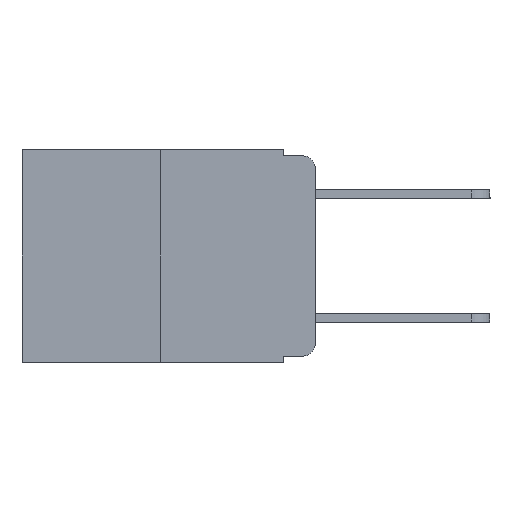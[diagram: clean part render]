
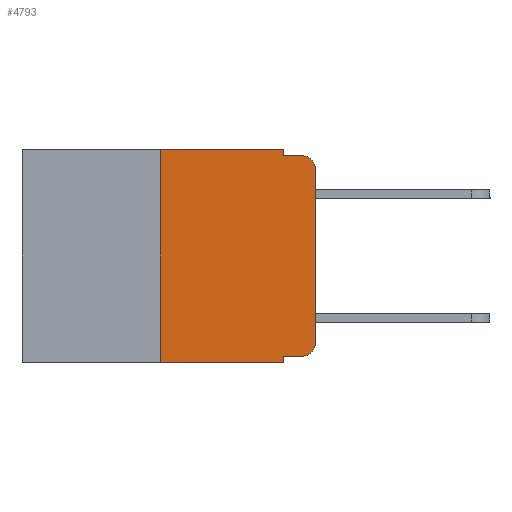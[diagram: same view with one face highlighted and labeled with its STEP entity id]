
A CAD part, left-side view. The second image highlights one B-rep face of the part: STEP entity #4793.
In plain terms, the highlighted planar face has unit normal (-1, 0, 0).
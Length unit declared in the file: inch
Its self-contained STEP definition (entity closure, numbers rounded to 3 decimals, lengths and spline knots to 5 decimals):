
#39 = VERTEX_POINT ( 'NONE', #19924 ) ;
#89 = CARTESIAN_POINT ( 'NONE',  ( 0., 0.473, 0. ) ) ;
#258 = CARTESIAN_POINT ( 'NONE',  ( 0., 0., -0.03 ) ) ;
#409 = PLANE ( 'NONE',  #3439 ) ;
#651 = CARTESIAN_POINT ( 'NONE',  ( 0., 0.473, 0. ) ) ;
#1153 = VERTEX_POINT ( 'NONE', #19772 ) ;
#1173 = ORIENTED_EDGE ( 'NONE', *, *, #15919, .F. ) ;
#1188 = VECTOR ( 'NONE', #7753, 39.37008 ) ;
#1391 = VERTEX_POINT ( 'NONE', #6716 ) ;
#1683 = DIRECTION ( 'NONE',  ( 0., 0., -1. ) ) ;
#2019 = VERTEX_POINT ( 'NONE', #19199 ) ;
#2076 = LINE ( 'NONE', #18464, #6867 ) ;
#2133 = CARTESIAN_POINT ( 'NONE',  ( 0., 0.051, 0. ) ) ;
#2309 = VECTOR ( 'NONE', #15139, 39.37008 ) ;
#2660 = CARTESIAN_POINT ( 'NONE',  ( 0., 0.051, -0.343 ) ) ;
#2833 = AXIS2_PLACEMENT_3D ( 'NONE', #19030, #16500, #13619 ) ;
#2994 = EDGE_CURVE ( 'NONE', #5129, #16042, #19267, .T. ) ;
#3151 = ORIENTED_EDGE ( 'NONE', *, *, #11706, .T. ) ;
#3439 = AXIS2_PLACEMENT_3D ( 'NONE', #651, #14961, #15179 ) ;
#3998 = DIRECTION ( 'NONE',  ( 0., 0., 1. ) ) ;
#4396 = CIRCLE ( 'NONE', #2833, 0.02 ) ;
#4793 = ADVANCED_FACE ( 'NONE', ( #16140 ), #409, .F. ) ;
#5129 = VERTEX_POINT ( 'NONE', #17437 ) ;
#5577 = EDGE_CURVE ( 'NONE', #16042, #1391, #4396, .T. ) ;
#5991 = ORIENTED_EDGE ( 'NONE', *, *, #16805, .T. ) ;
#6115 = EDGE_CURVE ( 'NONE', #1153, #1391, #2076, .T. ) ;
#6242 = EDGE_CURVE ( 'NONE', #16015, #1153, #15265, .T. ) ;
#6550 = CARTESIAN_POINT ( 'NONE',  ( 0., 0.02, -0.313 ) ) ;
#6612 = VECTOR ( 'NONE', #8444, 39.37008 ) ;
#6716 = CARTESIAN_POINT ( 'NONE',  ( 0., 0.02, -0.01 ) ) ;
#6867 = VECTOR ( 'NONE', #13075, 39.37008 ) ;
#6942 = EDGE_CURVE ( 'NONE', #39, #17255, #12113, .T. ) ;
#7401 = CARTESIAN_POINT ( 'NONE',  ( 0., 0.051, 0. ) ) ;
#7753 = DIRECTION ( 'NONE',  ( 0., -1., 0. ) ) ;
#7913 = CARTESIAN_POINT ( 'NONE',  ( 0., 0.051, 0. ) ) ;
#8070 = VERTEX_POINT ( 'NONE', #2660 ) ;
#8177 = LINE ( 'NONE', #2133, #2309 ) ;
#8303 = DIRECTION ( 'NONE',  ( 0., 0., -1. ) ) ;
#8444 = DIRECTION ( 'NONE',  ( 0., -1., 0. ) ) ;
#8797 = CARTESIAN_POINT ( 'NONE',  ( 0., 0.25, 0. ) ) ;
#9285 = ORIENTED_EDGE ( 'NONE', *, *, #13849, .F. ) ;
#10081 = EDGE_LOOP ( 'NONE', ( #10996, #11683, #13234, #11010, #1173, #15646, #3151, #9285, #12124, #5991 ) ) ;
#10996 = ORIENTED_EDGE ( 'NONE', *, *, #2994, .T. ) ;
#11010 = ORIENTED_EDGE ( 'NONE', *, *, #6242, .F. ) ;
#11079 = LINE ( 'NONE', #14479, #6612 ) ;
#11495 = VECTOR ( 'NONE', #1683, 39.37008 ) ;
#11683 = ORIENTED_EDGE ( 'NONE', *, *, #5577, .T. ) ;
#11706 = EDGE_CURVE ( 'NONE', #39, #8070, #11079, .T. ) ;
#12113 = LINE ( 'NONE', #8797, #15831 ) ;
#12124 = ORIENTED_EDGE ( 'NONE', *, *, #13956, .T. ) ;
#12530 = CARTESIAN_POINT ( 'NONE',  ( 0., 0.051, -0.333 ) ) ;
#12964 = VECTOR ( 'NONE', #14977, 39.37008 ) ;
#13075 = DIRECTION ( 'NONE',  ( 0., -1., 0. ) ) ;
#13234 = ORIENTED_EDGE ( 'NONE', *, *, #6115, .F. ) ;
#13612 = CARTESIAN_POINT ( 'NONE',  ( 0., 0.25, 0. ) ) ;
#13619 = DIRECTION ( 'NONE',  ( 0., 0., -1. ) ) ;
#13849 = EDGE_CURVE ( 'NONE', #2019, #8070, #8177, .T. ) ;
#13956 = EDGE_CURVE ( 'NONE', #2019, #18434, #16667, .T. ) ;
#14479 = CARTESIAN_POINT ( 'NONE',  ( 0., 0.473, -0.343 ) ) ;
#14961 = DIRECTION ( 'NONE',  ( 1., 0., 0. ) ) ;
#14977 = DIRECTION ( 'NONE',  ( 0., -1., 0. ) ) ;
#14979 = AXIS2_PLACEMENT_3D ( 'NONE', #6550, #17016, #8303 ) ;
#15139 = DIRECTION ( 'NONE',  ( 0., 0., -1. ) ) ;
#15179 = DIRECTION ( 'NONE',  ( 0., 0., -1. ) ) ;
#15265 = LINE ( 'NONE', #7913, #11495 ) ;
#15646 = ORIENTED_EDGE ( 'NONE', *, *, #6942, .F. ) ;
#15831 = VECTOR ( 'NONE', #18707, 39.37008 ) ;
#15919 = EDGE_CURVE ( 'NONE', #17255, #16015, #17020, .T. ) ;
#16015 = VERTEX_POINT ( 'NONE', #7401 ) ;
#16042 = VERTEX_POINT ( 'NONE', #258 ) ;
#16140 = FACE_OUTER_BOUND ( 'NONE', #10081, .T. ) ;
#16500 = DIRECTION ( 'NONE',  ( -1., 0., 0. ) ) ;
#16667 = LINE ( 'NONE', #12530, #1188 ) ;
#16805 = EDGE_CURVE ( 'NONE', #18434, #5129, #18240, .T. ) ;
#17016 = DIRECTION ( 'NONE',  ( -1., 0., 0. ) ) ;
#17020 = LINE ( 'NONE', #89, #12964 ) ;
#17255 = VERTEX_POINT ( 'NONE', #13612 ) ;
#17437 = CARTESIAN_POINT ( 'NONE',  ( 0., 0., -0.313 ) ) ;
#17694 = CARTESIAN_POINT ( 'NONE',  ( 0., 0., 0. ) ) ;
#18240 = CIRCLE ( 'NONE', #14979, 0.02 ) ;
#18434 = VERTEX_POINT ( 'NONE', #18986 ) ;
#18464 = CARTESIAN_POINT ( 'NONE',  ( 0., 0.051, -0.01 ) ) ;
#18707 = DIRECTION ( 'NONE',  ( 0., 0., 1. ) ) ;
#18876 = VECTOR ( 'NONE', #3998, 39.37008 ) ;
#18986 = CARTESIAN_POINT ( 'NONE',  ( 0., 0.02, -0.333 ) ) ;
#19030 = CARTESIAN_POINT ( 'NONE',  ( 0., 0.02, -0.03 ) ) ;
#19199 = CARTESIAN_POINT ( 'NONE',  ( 0., 0.051, -0.333 ) ) ;
#19267 = LINE ( 'NONE', #17694, #18876 ) ;
#19772 = CARTESIAN_POINT ( 'NONE',  ( 0., 0.051, -0.01 ) ) ;
#19924 = CARTESIAN_POINT ( 'NONE',  ( 0., 0.25, -0.343 ) ) ;
